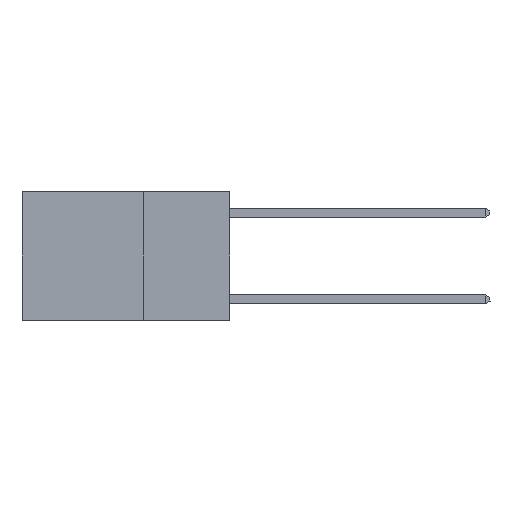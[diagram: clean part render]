
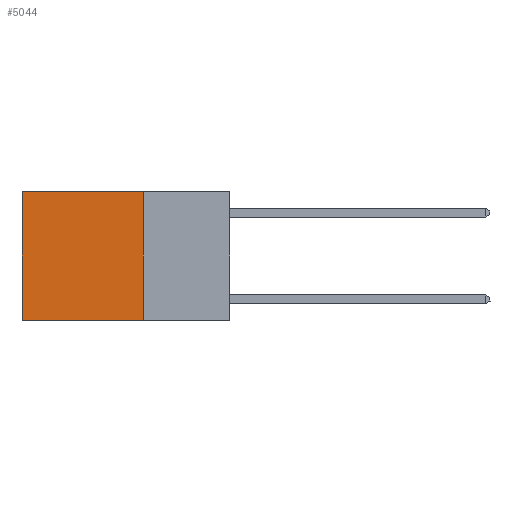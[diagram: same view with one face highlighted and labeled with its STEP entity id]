
A CAD part, left-side view. The second image highlights one B-rep face of the part: STEP entity #5044.
In plain terms, the highlighted planar face has unit normal (-1, 0, 0).
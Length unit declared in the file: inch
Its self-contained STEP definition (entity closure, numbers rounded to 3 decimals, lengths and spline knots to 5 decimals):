
#220 = VECTOR ( 'NONE', #9397, 39.37008 ) ;
#231 = ORIENTED_EDGE ( 'NONE', *, *, #9852, .T. ) ;
#233 = CARTESIAN_POINT ( 'NONE',  ( 0.2625, 0.6, -0.37 ) ) ;
#695 = EDGE_LOOP ( 'NONE', ( #7500, #3697, #4125, #231 ) ) ;
#860 = VECTOR ( 'NONE', #5006, 39.37008 ) ;
#1314 = VERTEX_POINT ( 'NONE', #10247 ) ;
#1558 = LINE ( 'NONE', #13372, #860 ) ;
#2324 = CARTESIAN_POINT ( 'NONE',  ( 0.2625, 0.6, 0. ) ) ;
#3463 = DIRECTION ( 'NONE',  ( 0., 0., -1. ) ) ;
#3526 = CARTESIAN_POINT ( 'NONE',  ( 0.2625, 0.25, 0. ) ) ;
#3559 = EDGE_CURVE ( 'NONE', #6804, #8129, #12032, .T. ) ;
#3697 = ORIENTED_EDGE ( 'NONE', *, *, #13154, .F. ) ;
#4125 = ORIENTED_EDGE ( 'NONE', *, *, #11414, .F. ) ;
#4619 = CARTESIAN_POINT ( 'NONE',  ( 0.2625, 0.6, 0. ) ) ;
#4717 = DIRECTION ( 'NONE',  ( 0., 0., -1. ) ) ;
#5006 = DIRECTION ( 'NONE',  ( 0., 1., 0. ) ) ;
#5044 = ADVANCED_FACE ( 'NONE', ( #10005 ), #8984, .F. ) ;
#5813 = DIRECTION ( 'NONE',  ( 0., 0., -1. ) ) ;
#6804 = VERTEX_POINT ( 'NONE', #4619 ) ;
#6834 = VERTEX_POINT ( 'NONE', #3526 ) ;
#6898 = CARTESIAN_POINT ( 'NONE',  ( 0.2625, 0.25, 0. ) ) ;
#7500 = ORIENTED_EDGE ( 'NONE', *, *, #3559, .T. ) ;
#7963 = LINE ( 'NONE', #6898, #12471 ) ;
#8129 = VERTEX_POINT ( 'NONE', #233 ) ;
#8967 = VECTOR ( 'NONE', #3463, 39.37008 ) ;
#8984 = PLANE ( 'NONE',  #9906 ) ;
#9397 = DIRECTION ( 'NONE',  ( 0., 1., 0. ) ) ;
#9852 = EDGE_CURVE ( 'NONE', #6834, #6804, #1558, .T. ) ;
#9906 = AXIS2_PLACEMENT_3D ( 'NONE', #9998, #11034, #4717 ) ;
#9998 = CARTESIAN_POINT ( 'NONE',  ( 0.2625, 0.25, 0. ) ) ;
#10005 = FACE_OUTER_BOUND ( 'NONE', #695, .T. ) ;
#10247 = CARTESIAN_POINT ( 'NONE',  ( 0.2625, 0.25, -0.37 ) ) ;
#11034 = DIRECTION ( 'NONE',  ( 1., 0., 0. ) ) ;
#11414 = EDGE_CURVE ( 'NONE', #6834, #1314, #7963, .T. ) ;
#11755 = LINE ( 'NONE', #13511, #220 ) ;
#12032 = LINE ( 'NONE', #2324, #8967 ) ;
#12471 = VECTOR ( 'NONE', #5813, 39.37008 ) ;
#13154 = EDGE_CURVE ( 'NONE', #1314, #8129, #11755, .T. ) ;
#13372 = CARTESIAN_POINT ( 'NONE',  ( 0.2625, 0.25, 0. ) ) ;
#13511 = CARTESIAN_POINT ( 'NONE',  ( 0.2625, 0.25, -0.37 ) ) ;
